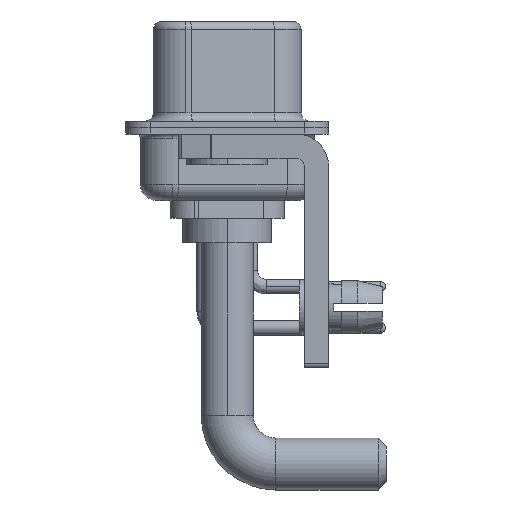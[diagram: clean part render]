
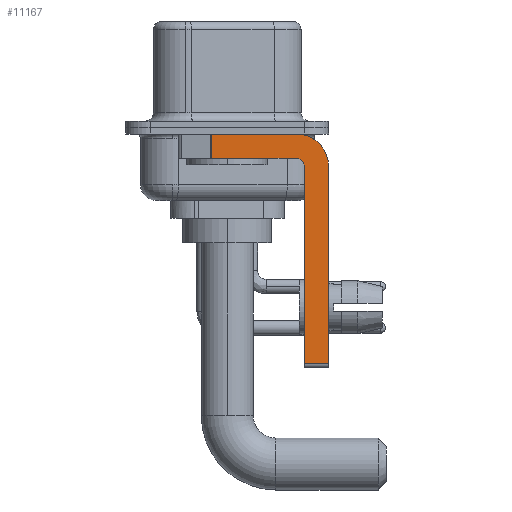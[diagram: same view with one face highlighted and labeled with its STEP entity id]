
A CAD part, left-side view. The second image highlights one B-rep face of the part: STEP entity #11167.
In plain terms, the highlighted planar face has unit normal (-1, 0, 0).
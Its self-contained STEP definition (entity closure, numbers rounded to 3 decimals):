
#210 = LINE ( 'NONE', #18918, #21782 ) ;
#257 = VECTOR ( 'NONE', #9093, 1000. ) ;
#559 = ORIENTED_EDGE ( 'NONE', *, *, #5431, .F. ) ;
#1685 = AXIS2_PLACEMENT_3D ( 'NONE', #2263, #18341, #6872 ) ;
#1940 = CARTESIAN_POINT ( 'NONE',  ( -2.9, 3., -0.4 ) ) ;
#2263 = CARTESIAN_POINT ( 'NONE',  ( -2.9, -4.25, -2.4 ) ) ;
#2369 = DIRECTION ( 'NONE',  ( -1., 0., 0. ) ) ;
#2511 = VERTEX_POINT ( 'NONE', #22434 ) ;
#3153 = CARTESIAN_POINT ( 'NONE',  ( -2.9, -6.25, -2.4 ) ) ;
#3186 = EDGE_CURVE ( 'NONE', #12130, #5562, #20431, .T. ) ;
#3978 = CARTESIAN_POINT ( 'NONE',  ( -2.9, -4.25, -1.9 ) ) ;
#4460 = LINE ( 'NONE', #18401, #11169 ) ;
#5127 = CIRCLE ( 'NONE', #1685, 2. ) ;
#5431 = EDGE_CURVE ( 'NONE', #2511, #9633, #27376, .T. ) ;
#5562 = VERTEX_POINT ( 'NONE', #9293 ) ;
#5692 = VECTOR ( 'NONE', #10019, 1000. ) ;
#6154 = VERTEX_POINT ( 'NONE', #3978 ) ;
#6872 = DIRECTION ( 'NONE',  ( 0., 0., -1. ) ) ;
#7436 = DIRECTION ( 'NONE',  ( 0., 0., 1. ) ) ;
#7739 = PLANE ( 'NONE',  #29234 ) ;
#7762 = DIRECTION ( 'NONE',  ( 0., 1., 0. ) ) ;
#7808 = ORIENTED_EDGE ( 'NONE', *, *, #11443, .T. ) ;
#8200 = EDGE_CURVE ( 'NONE', #9633, #12130, #5127, .T. ) ;
#9093 = DIRECTION ( 'NONE',  ( 0., 0., -1. ) ) ;
#9293 = CARTESIAN_POINT ( 'NONE',  ( -2.9, -6.25, -14.55 ) ) ;
#9633 = VERTEX_POINT ( 'NONE', #11260 ) ;
#9640 = AXIS2_PLACEMENT_3D ( 'NONE', #28262, #2369, #7436 ) ;
#9725 = LINE ( 'NONE', #23810, #5692 ) ;
#9738 = EDGE_CURVE ( 'NONE', #27293, #16204, #9725, .T. ) ;
#10019 = DIRECTION ( 'NONE',  ( 0., 0., 1. ) ) ;
#10238 = EDGE_CURVE ( 'NONE', #27293, #5562, #19024, .T. ) ;
#10261 = CARTESIAN_POINT ( 'NONE',  ( -2.9, 0.978, -1.9 ) ) ;
#11167 = ADVANCED_FACE ( 'NONE', ( #21504 ), #7739, .F. ) ;
#11169 = VECTOR ( 'NONE', #25448, 1000. ) ;
#11260 = CARTESIAN_POINT ( 'NONE',  ( -2.9, -4.25, -0.4 ) ) ;
#11443 = EDGE_CURVE ( 'NONE', #2511, #27461, #4460, .T. ) ;
#12130 = VERTEX_POINT ( 'NONE', #3153 ) ;
#12870 = ORIENTED_EDGE ( 'NONE', *, *, #25300, .F. ) ;
#13547 = VECTOR ( 'NONE', #23931, 1000. ) ;
#14424 = CARTESIAN_POINT ( 'NONE',  ( -2.9, -4.25, -14.55 ) ) ;
#15688 = ORIENTED_EDGE ( 'NONE', *, *, #26424, .F. ) ;
#16204 = VERTEX_POINT ( 'NONE', #29330 ) ;
#16537 = CARTESIAN_POINT ( 'NONE',  ( -2.9, -4.75, -14.55 ) ) ;
#16756 = DIRECTION ( 'NONE',  ( 1., 0., 0. ) ) ;
#18341 = DIRECTION ( 'NONE',  ( 1., 0., 0. ) ) ;
#18401 = CARTESIAN_POINT ( 'NONE',  ( -2.9, 0.978, -1.9 ) ) ;
#18918 = CARTESIAN_POINT ( 'NONE',  ( -2.9, -4.25, -1.9 ) ) ;
#19024 = LINE ( 'NONE', #14424, #13547 ) ;
#19389 = ORIENTED_EDGE ( 'NONE', *, *, #3186, .F. ) ;
#19511 = CARTESIAN_POINT ( 'NONE',  ( -2.9, -4.25, -2.4 ) ) ;
#20431 = LINE ( 'NONE', #25621, #257 ) ;
#20619 = DIRECTION ( 'NONE',  ( 0., -1., 0. ) ) ;
#20880 = CIRCLE ( 'NONE', #9640, 0.5 ) ;
#21504 = FACE_OUTER_BOUND ( 'NONE', #22531, .T. ) ;
#21782 = VECTOR ( 'NONE', #7762, 1000. ) ;
#22434 = CARTESIAN_POINT ( 'NONE',  ( -2.9, 0.978, -0.4 ) ) ;
#22531 = EDGE_LOOP ( 'NONE', ( #559, #7808, #12870, #15688, #28707, #29918, #19389, #29944 ) ) ;
#23810 = CARTESIAN_POINT ( 'NONE',  ( -2.9, -4.75, -14.8 ) ) ;
#23931 = DIRECTION ( 'NONE',  ( 0., -1., 0. ) ) ;
#25300 = EDGE_CURVE ( 'NONE', #6154, #27461, #210, .T. ) ;
#25448 = DIRECTION ( 'NONE',  ( 0., 0., -1. ) ) ;
#25621 = CARTESIAN_POINT ( 'NONE',  ( -2.9, -6.25, -2.4 ) ) ;
#26424 = EDGE_CURVE ( 'NONE', #16204, #6154, #20880, .T. ) ;
#27293 = VERTEX_POINT ( 'NONE', #16537 ) ;
#27376 = LINE ( 'NONE', #1940, #28699 ) ;
#27461 = VERTEX_POINT ( 'NONE', #10261 ) ;
#28262 = CARTESIAN_POINT ( 'NONE',  ( -2.9, -4.25, -2.4 ) ) ;
#28699 = VECTOR ( 'NONE', #20619, 1000. ) ;
#28707 = ORIENTED_EDGE ( 'NONE', *, *, #9738, .F. ) ;
#28711 = DIRECTION ( 'NONE',  ( 0., 0., -1. ) ) ;
#29234 = AXIS2_PLACEMENT_3D ( 'NONE', #19511, #16756, #28711 ) ;
#29330 = CARTESIAN_POINT ( 'NONE',  ( -2.9, -4.75, -2.4 ) ) ;
#29918 = ORIENTED_EDGE ( 'NONE', *, *, #10238, .T. ) ;
#29944 = ORIENTED_EDGE ( 'NONE', *, *, #8200, .F. ) ;
